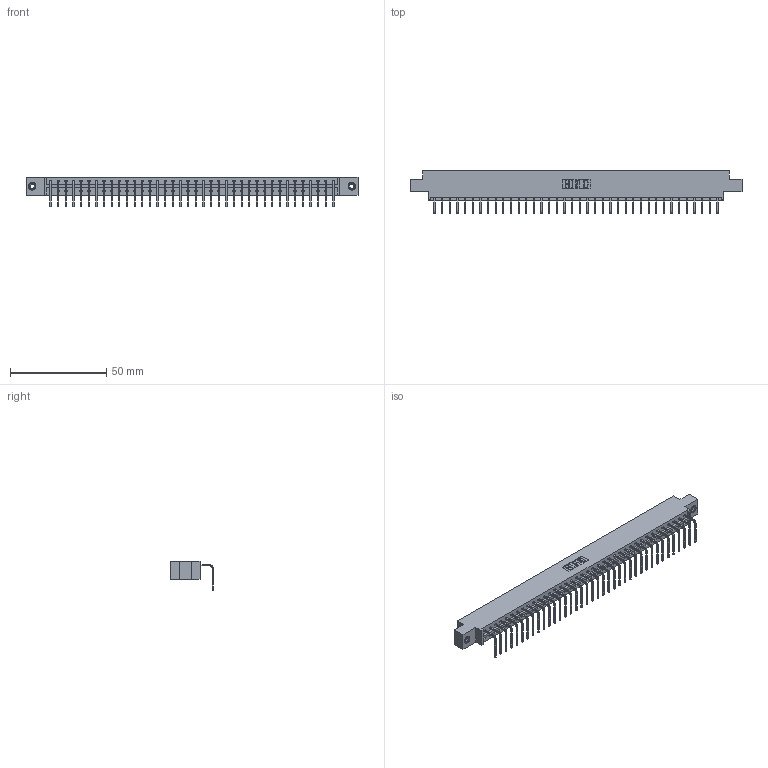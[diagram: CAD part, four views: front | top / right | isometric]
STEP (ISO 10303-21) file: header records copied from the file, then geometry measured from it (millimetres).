
FILE_DESCRIPTION (( 'STEP AP203' ), '1' );
FILE_NAME ('833-038-558-608.STEP', '2020-06-03T13:44:26', ( '' ), ( '' ), 'SwSTEP 2.0', 'SolidWorks 2020', '' );
FILE_SCHEMA (( 'CONFIG_CONTROL_DESIGN' ));
Length unit declared in the file: inch
Products named in the file (4): 345-250-001_345-250-003-102; 833-038-558-608; 833 Part_Offset - .156 Dia - TI; 345-292-001_558 Tail - 2
Assembly tree (41 placements, depth 2):
  833-038-558-608
    833 Part_Offset - .156 Dia - TI
    345-292-001_558 Tail - 2  x38
    345-250-001_345-250-003-102  x2
Bounding box: 172.11 x 22.17 x 15.37 mm (x, y, z)
Volume: 17177.1 mm3; surface area: 19559.3 mm2
Topology: 41 solids, 41 shells, 2458 faces, 7375 edges, 4858 vertices
Faces by surface type: plane 1778, cylinder 664, cone 12, torus 4
Entity records: 25150 total; most frequent: CARTESIAN_POINT 4323, ORIENTED_EDGE 4290, DIRECTION 3687, EDGE_CURVE 2145, VECTOR 1997, LINE 1997, VERTEX_POINT 1424, AXIS2_PLACEMENT_3D 845
